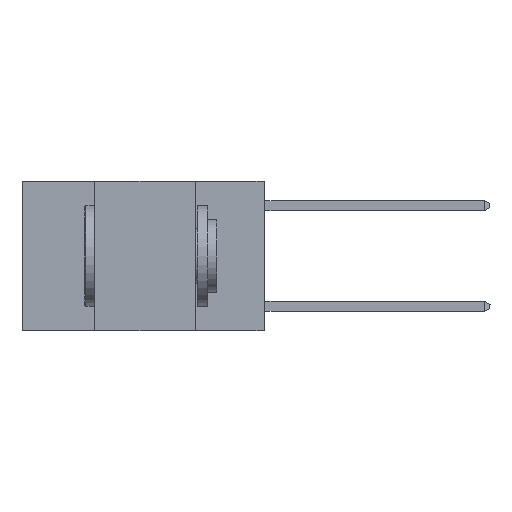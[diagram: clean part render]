
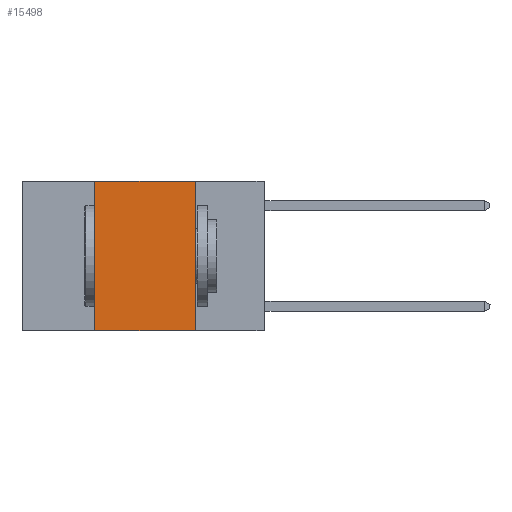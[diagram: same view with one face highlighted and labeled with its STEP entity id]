
A CAD part, left-side view. The second image highlights one B-rep face of the part: STEP entity #15498.
In plain terms, the highlighted planar face has unit normal (-1, 0, 0).
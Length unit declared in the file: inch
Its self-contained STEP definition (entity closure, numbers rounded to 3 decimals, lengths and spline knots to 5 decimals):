
#751 = VERTEX_POINT ( 'NONE', #15886 ) ;
#922 = DIRECTION ( 'NONE',  ( 0., 0., 1. ) ) ;
#1156 = DIRECTION ( 'NONE',  ( 0., -1., 0. ) ) ;
#1164 = VECTOR ( 'NONE', #922, 39.37008 ) ;
#1245 = EDGE_CURVE ( 'NONE', #8387, #751, #14629, .T. ) ;
#3705 = LINE ( 'NONE', #6590, #18120 ) ;
#4105 = EDGE_LOOP ( 'NONE', ( #15492, #9137, #15192, #6054 ) ) ;
#4139 = CARTESIAN_POINT ( 'NONE',  ( 0., 0.6, -0.37 ) ) ;
#4499 = PLANE ( 'NONE',  #17912 ) ;
#5166 = LINE ( 'NONE', #5409, #1164 ) ;
#5193 = DIRECTION ( 'NONE',  ( 0., 0., -1. ) ) ;
#5409 = CARTESIAN_POINT ( 'NONE',  ( 0., 0.42, 0. ) ) ;
#6054 = ORIENTED_EDGE ( 'NONE', *, *, #11534, .T. ) ;
#6590 = CARTESIAN_POINT ( 'NONE',  ( 0., 0.17, 0. ) ) ;
#6659 = CARTESIAN_POINT ( 'NONE',  ( 0., 0.17, -0.37 ) ) ;
#8387 = VERTEX_POINT ( 'NONE', #17972 ) ;
#8548 = VECTOR ( 'NONE', #17058, 39.37008 ) ;
#8792 = DIRECTION ( 'NONE',  ( 1., 0., 0. ) ) ;
#9137 = ORIENTED_EDGE ( 'NONE', *, *, #1245, .F. ) ;
#10566 = EDGE_CURVE ( 'NONE', #751, #12866, #3705, .T. ) ;
#11244 = CARTESIAN_POINT ( 'NONE',  ( 0., 0.42, -0.37 ) ) ;
#11534 = EDGE_CURVE ( 'NONE', #16180, #12866, #15849, .T. ) ;
#12224 = VECTOR ( 'NONE', #1156, 39.37008 ) ;
#12866 = VERTEX_POINT ( 'NONE', #6659 ) ;
#14629 = LINE ( 'NONE', #17380, #8548 ) ;
#15192 = ORIENTED_EDGE ( 'NONE', *, *, #15232, .F. ) ;
#15232 = EDGE_CURVE ( 'NONE', #16180, #8387, #5166, .T. ) ;
#15492 = ORIENTED_EDGE ( 'NONE', *, *, #10566, .F. ) ;
#15498 = ADVANCED_FACE ( 'NONE', ( #17765 ), #4499, .F. ) ;
#15849 = LINE ( 'NONE', #4139, #12224 ) ;
#15886 = CARTESIAN_POINT ( 'NONE',  ( 0., 0.17, 0. ) ) ;
#16180 = VERTEX_POINT ( 'NONE', #11244 ) ;
#16985 = CARTESIAN_POINT ( 'NONE',  ( 0., 0.6, 0. ) ) ;
#17058 = DIRECTION ( 'NONE',  ( 0., -1., 0. ) ) ;
#17380 = CARTESIAN_POINT ( 'NONE',  ( 0., 0.6, 0. ) ) ;
#17765 = FACE_OUTER_BOUND ( 'NONE', #4105, .T. ) ;
#17912 = AXIS2_PLACEMENT_3D ( 'NONE', #16985, #8792, #18286 ) ;
#17972 = CARTESIAN_POINT ( 'NONE',  ( 0., 0.42, 0. ) ) ;
#18120 = VECTOR ( 'NONE', #5193, 39.37008 ) ;
#18286 = DIRECTION ( 'NONE',  ( 0., 0., -1. ) ) ;
